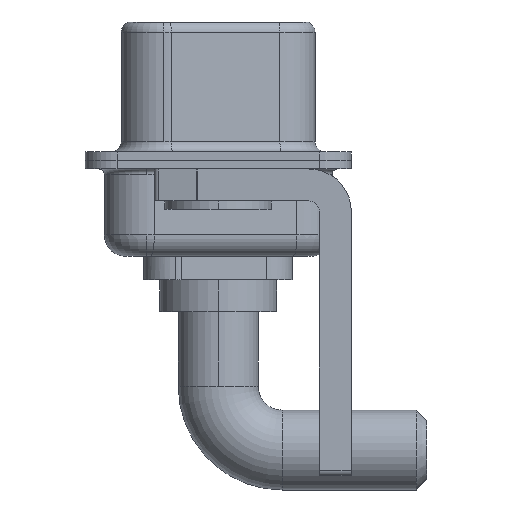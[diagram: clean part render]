
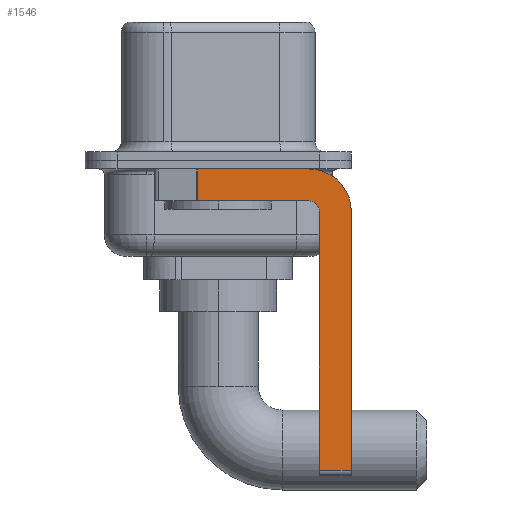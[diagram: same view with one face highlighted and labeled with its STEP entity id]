
A CAD part, left-side view. The second image highlights one B-rep face of the part: STEP entity #1546.
In plain terms, the highlighted planar face has unit normal (-1, 0, 0).
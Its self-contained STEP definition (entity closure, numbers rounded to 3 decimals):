
#187 = DIRECTION ( 'NONE',  ( 0., 0., -1. ) ) ;
#1546 = ADVANCED_FACE ( 'NONE', ( #9553 ), #3480, .F. ) ;
#1697 = VERTEX_POINT ( 'NONE', #15294 ) ;
#1886 = DIRECTION ( 'NONE',  ( 0., 0., 1. ) ) ;
#2139 = CARTESIAN_POINT ( 'NONE',  ( -2.9, -4.25, -1.9 ) ) ;
#2164 = EDGE_CURVE ( 'NONE', #12240, #12892, #12692, .T. ) ;
#2866 = EDGE_CURVE ( 'NONE', #7638, #4461, #9319, .T. ) ;
#2937 = ORIENTED_EDGE ( 'NONE', *, *, #2866, .F. ) ;
#2969 = EDGE_CURVE ( 'NONE', #11700, #1697, #3225, .T. ) ;
#3225 = LINE ( 'NONE', #2139, #10934 ) ;
#3231 = VECTOR ( 'NONE', #7337, 1000. ) ;
#3480 = PLANE ( 'NONE',  #10369 ) ;
#3632 = CIRCLE ( 'NONE', #15322, 2. ) ;
#3913 = CIRCLE ( 'NONE', #8160, 0.5 ) ;
#4011 = DIRECTION ( 'NONE',  ( 0., 0., -1. ) ) ;
#4061 = ORIENTED_EDGE ( 'NONE', *, *, #10036, .F. ) ;
#4461 = VERTEX_POINT ( 'NONE', #13783 ) ;
#4788 = CARTESIAN_POINT ( 'NONE',  ( -2.9, -4.25, -1.9 ) ) ;
#4814 = EDGE_CURVE ( 'NONE', #7638, #12892, #7174, .T. ) ;
#5615 = LINE ( 'NONE', #6725, #10732 ) ;
#5875 = VECTOR ( 'NONE', #1886, 1000. ) ;
#6142 = VECTOR ( 'NONE', #4011, 1000. ) ;
#6264 = ORIENTED_EDGE ( 'NONE', *, *, #2969, .F. ) ;
#6311 = CARTESIAN_POINT ( 'NONE',  ( -2.9, 0.978, -0.4 ) ) ;
#6528 = CARTESIAN_POINT ( 'NONE',  ( -2.9, -4.25, -2.4 ) ) ;
#6725 = CARTESIAN_POINT ( 'NONE',  ( -2.9, 0.978, -1.9 ) ) ;
#6956 = EDGE_CURVE ( 'NONE', #9833, #1697, #5615, .T. ) ;
#7174 = LINE ( 'NONE', #11158, #3231 ) ;
#7335 = ORIENTED_EDGE ( 'NONE', *, *, #2164, .F. ) ;
#7337 = DIRECTION ( 'NONE',  ( 0., -1., 0. ) ) ;
#7638 = VERTEX_POINT ( 'NONE', #14314 ) ;
#7888 = CARTESIAN_POINT ( 'NONE',  ( -2.9, 3., -0.4 ) ) ;
#7921 = CARTESIAN_POINT ( 'NONE',  ( -2.9, -6.25, -14.55 ) ) ;
#8160 = AXIS2_PLACEMENT_3D ( 'NONE', #15439, #11459, #14274 ) ;
#8556 = DIRECTION ( 'NONE',  ( 0., 0., -1. ) ) ;
#9193 = ORIENTED_EDGE ( 'NONE', *, *, #14935, .F. ) ;
#9319 = LINE ( 'NONE', #9476, #5875 ) ;
#9476 = CARTESIAN_POINT ( 'NONE',  ( -2.9, -4.75, -14.8 ) ) ;
#9553 = FACE_OUTER_BOUND ( 'NONE', #10850, .T. ) ;
#9833 = VERTEX_POINT ( 'NONE', #6311 ) ;
#10036 = EDGE_CURVE ( 'NONE', #4461, #11700, #3913, .T. ) ;
#10369 = AXIS2_PLACEMENT_3D ( 'NONE', #12227, #15957, #8556 ) ;
#10516 = EDGE_CURVE ( 'NONE', #14091, #12240, #3632, .T. ) ;
#10732 = VECTOR ( 'NONE', #11796, 1000. ) ;
#10850 = EDGE_LOOP ( 'NONE', ( #9193, #16388, #6264, #4061, #2937, #15869, #7335, #11318 ) ) ;
#10934 = VECTOR ( 'NONE', #16044, 1000. ) ;
#11158 = CARTESIAN_POINT ( 'NONE',  ( -2.9, -4.25, -14.55 ) ) ;
#11318 = ORIENTED_EDGE ( 'NONE', *, *, #10516, .F. ) ;
#11395 = LINE ( 'NONE', #7888, #12653 ) ;
#11459 = DIRECTION ( 'NONE',  ( -1., 0., 0. ) ) ;
#11600 = DIRECTION ( 'NONE',  ( 1., 0., 0. ) ) ;
#11700 = VERTEX_POINT ( 'NONE', #4788 ) ;
#11796 = DIRECTION ( 'NONE',  ( 0., 0., -1. ) ) ;
#12227 = CARTESIAN_POINT ( 'NONE',  ( -2.9, -4.25, -2.4 ) ) ;
#12240 = VERTEX_POINT ( 'NONE', #16266 ) ;
#12653 = VECTOR ( 'NONE', #16461, 1000. ) ;
#12692 = LINE ( 'NONE', #14011, #6142 ) ;
#12892 = VERTEX_POINT ( 'NONE', #7921 ) ;
#13783 = CARTESIAN_POINT ( 'NONE',  ( -2.9, -4.75, -2.4 ) ) ;
#14011 = CARTESIAN_POINT ( 'NONE',  ( -2.9, -6.25, -2.4 ) ) ;
#14091 = VERTEX_POINT ( 'NONE', #15240 ) ;
#14274 = DIRECTION ( 'NONE',  ( 0., 0., 1. ) ) ;
#14314 = CARTESIAN_POINT ( 'NONE',  ( -2.9, -4.75, -14.55 ) ) ;
#14935 = EDGE_CURVE ( 'NONE', #9833, #14091, #11395, .T. ) ;
#15240 = CARTESIAN_POINT ( 'NONE',  ( -2.9, -4.25, -0.4 ) ) ;
#15294 = CARTESIAN_POINT ( 'NONE',  ( -2.9, 0.978, -1.9 ) ) ;
#15322 = AXIS2_PLACEMENT_3D ( 'NONE', #6528, #11600, #187 ) ;
#15439 = CARTESIAN_POINT ( 'NONE',  ( -2.9, -4.25, -2.4 ) ) ;
#15869 = ORIENTED_EDGE ( 'NONE', *, *, #4814, .T. ) ;
#15957 = DIRECTION ( 'NONE',  ( 1., 0., 0. ) ) ;
#16044 = DIRECTION ( 'NONE',  ( 0., 1., 0. ) ) ;
#16266 = CARTESIAN_POINT ( 'NONE',  ( -2.9, -6.25, -2.4 ) ) ;
#16388 = ORIENTED_EDGE ( 'NONE', *, *, #6956, .T. ) ;
#16461 = DIRECTION ( 'NONE',  ( 0., -1., 0. ) ) ;
